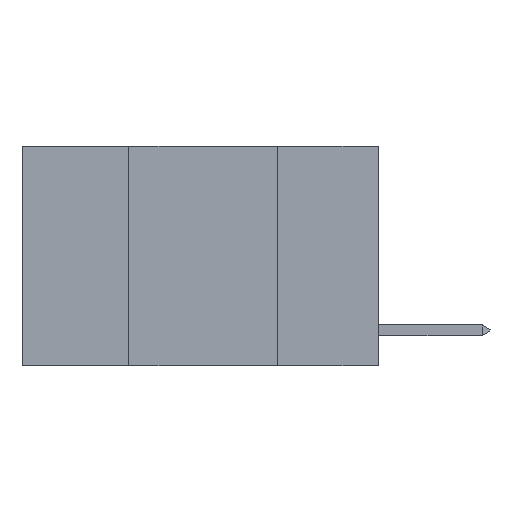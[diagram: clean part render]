
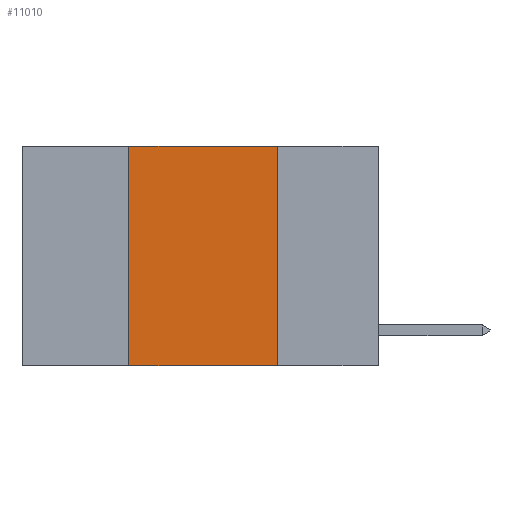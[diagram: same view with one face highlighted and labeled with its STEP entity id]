
A CAD part, left-side view. The second image highlights one B-rep face of the part: STEP entity #11010.
In plain terms, the highlighted planar face has unit normal (-1, 0, 0).
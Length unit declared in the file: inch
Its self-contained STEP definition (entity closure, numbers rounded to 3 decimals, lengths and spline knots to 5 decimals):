
#285 = CARTESIAN_POINT ( 'NONE',  ( 0., 0.17, -0.37 ) ) ;
#1756 = CARTESIAN_POINT ( 'NONE',  ( 0., 0.6, 0. ) ) ;
#2165 = VECTOR ( 'NONE', #6907, 39.37008 ) ;
#2317 = CARTESIAN_POINT ( 'NONE',  ( 0., 0.42, -0.37 ) ) ;
#2388 = DIRECTION ( 'NONE',  ( 0., 0., -1. ) ) ;
#3106 = VERTEX_POINT ( 'NONE', #9691 ) ;
#3360 = PLANE ( 'NONE',  #16463 ) ;
#3421 = EDGE_CURVE ( 'NONE', #9833, #16222, #4257, .T. ) ;
#3449 = CARTESIAN_POINT ( 'NONE',  ( 0., 0.42, 0. ) ) ;
#3538 = ORIENTED_EDGE ( 'NONE', *, *, #5132, .F. ) ;
#3666 = VERTEX_POINT ( 'NONE', #8249 ) ;
#4257 = LINE ( 'NONE', #9004, #7293 ) ;
#4372 = LINE ( 'NONE', #1756, #2165 ) ;
#4646 = DIRECTION ( 'NONE',  ( 0., 0., -1. ) ) ;
#5132 = EDGE_CURVE ( 'NONE', #9833, #3106, #5200, .T. ) ;
#5200 = LINE ( 'NONE', #3449, #15088 ) ;
#5497 = LINE ( 'NONE', #15234, #12356 ) ;
#6022 = DIRECTION ( 'NONE',  ( 0., 0., 1. ) ) ;
#6653 = FACE_OUTER_BOUND ( 'NONE', #15542, .T. ) ;
#6907 = DIRECTION ( 'NONE',  ( 0., -1., 0. ) ) ;
#7293 = VECTOR ( 'NONE', #11579, 39.37008 ) ;
#7454 = ORIENTED_EDGE ( 'NONE', *, *, #16270, .F. ) ;
#8249 = CARTESIAN_POINT ( 'NONE',  ( 0., 0.17, 0. ) ) ;
#8511 = ORIENTED_EDGE ( 'NONE', *, *, #12899, .F. ) ;
#9004 = CARTESIAN_POINT ( 'NONE',  ( 0., 0.6, -0.37 ) ) ;
#9691 = CARTESIAN_POINT ( 'NONE',  ( 0., 0.42, 0. ) ) ;
#9833 = VERTEX_POINT ( 'NONE', #2317 ) ;
#11000 = CARTESIAN_POINT ( 'NONE',  ( 0., 0.6, 0. ) ) ;
#11010 = ADVANCED_FACE ( 'NONE', ( #6653 ), #3360, .F. ) ;
#11579 = DIRECTION ( 'NONE',  ( 0., -1., 0. ) ) ;
#12346 = DIRECTION ( 'NONE',  ( 1., 0., 0. ) ) ;
#12356 = VECTOR ( 'NONE', #2388, 39.37008 ) ;
#12899 = EDGE_CURVE ( 'NONE', #3666, #16222, #5497, .T. ) ;
#15088 = VECTOR ( 'NONE', #6022, 39.37008 ) ;
#15234 = CARTESIAN_POINT ( 'NONE',  ( 0., 0.17, 0. ) ) ;
#15392 = ORIENTED_EDGE ( 'NONE', *, *, #3421, .T. ) ;
#15542 = EDGE_LOOP ( 'NONE', ( #8511, #7454, #3538, #15392 ) ) ;
#16222 = VERTEX_POINT ( 'NONE', #285 ) ;
#16270 = EDGE_CURVE ( 'NONE', #3106, #3666, #4372, .T. ) ;
#16463 = AXIS2_PLACEMENT_3D ( 'NONE', #11000, #12346, #4646 ) ;
